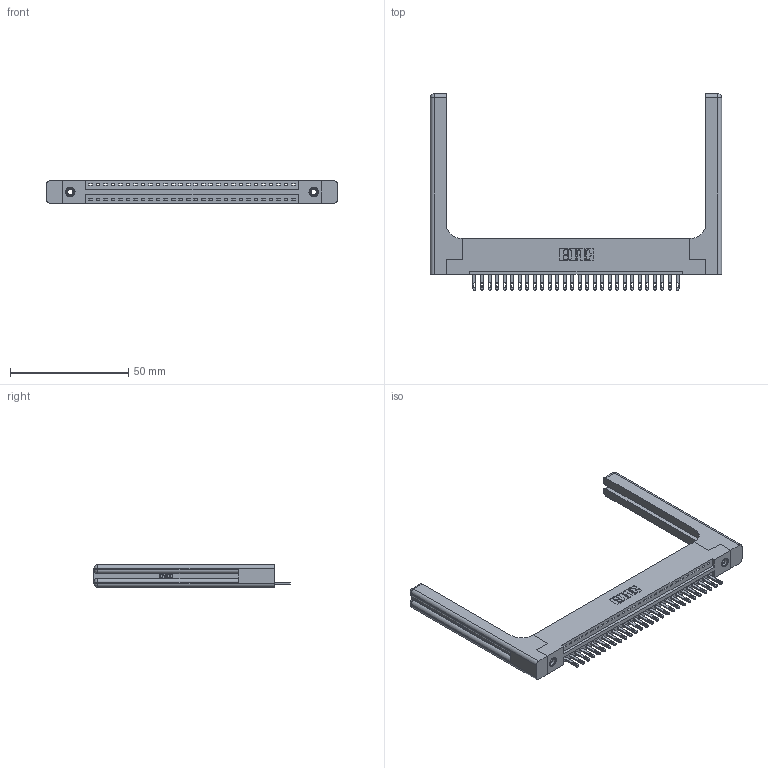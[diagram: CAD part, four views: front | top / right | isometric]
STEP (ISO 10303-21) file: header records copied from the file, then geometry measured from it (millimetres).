
FILE_DESCRIPTION (( 'STEP AP203' ), '1' );
FILE_NAME ('346-028-500-158.STEP', '2022-05-06T05:58:39', ( '' ), ( '' ), 'SwSTEP 2.0', 'SolidWorks 2020', '' );
FILE_SCHEMA (( 'CONFIG_CONTROL_DESIGN' ));
Length unit declared in the file: inch
Products named in the file (5): 345-292-001_345-293-100; 346 Part_Flush Mounting Lugs - 0.156 Dia-TH; 345-250-001_345-250-001-102; 346-220-058_345-220-058; 346-028-500-158
Assembly tree (33 placements, depth 2):
  346-028-500-158
    346 Part_Flush Mounting Lugs - 0.156 Dia-TH
    345-292-001_345-293-100  x28
    345-250-001_345-250-001-102  x2
    346-220-058_345-220-058  x2
Bounding box: 122.96 x 82.8 x 9.4 mm (x, y, z)
Volume: 19191.3 mm3; surface area: 19705.6 mm2
Topology: 33 solids, 33 shells, 1904 faces, 5735 edges, 3802 vertices
Faces by surface type: plane 1190, cylinder 654, bspline 36, cone 12, sphere 8, torus 4
Entity records: 24790 total; most frequent: CARTESIAN_POINT 5235, ORIENTED_EDGE 3992, DIRECTION 3568, EDGE_CURVE 1996, LINE 1656, VECTOR 1656, VERTEX_POINT 1322, AXIS2_PLACEMENT_3D 956
